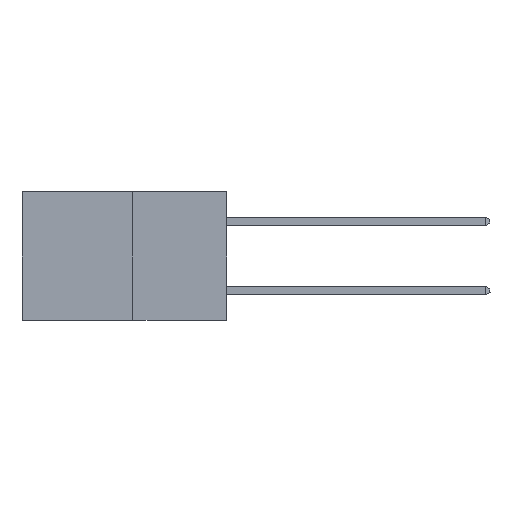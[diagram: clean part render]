
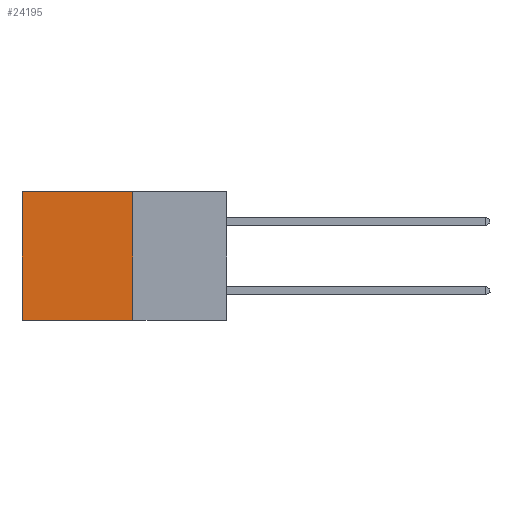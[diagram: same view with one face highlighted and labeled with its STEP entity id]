
A CAD part, left-side view. The second image highlights one B-rep face of the part: STEP entity #24195.
In plain terms, the highlighted planar face has unit normal (-1, 0, 0).
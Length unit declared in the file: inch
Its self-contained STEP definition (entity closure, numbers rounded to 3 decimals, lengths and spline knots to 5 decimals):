
#1287 = DIRECTION ( 'NONE',  ( 0., 0., -1. ) ) ;
#1591 = LINE ( 'NONE', #22627, #19816 ) ;
#2851 = CARTESIAN_POINT ( 'NONE',  ( 0.277, 0.59, -0.37 ) ) ;
#3229 = ORIENTED_EDGE ( 'NONE', *, *, #11312, .T. ) ;
#4168 = EDGE_CURVE ( 'NONE', #6265, #18495, #6261, .T. ) ;
#4348 = VECTOR ( 'NONE', #26284, 39.37008 ) ;
#5736 = EDGE_CURVE ( 'NONE', #10823, #8183, #19189, .T. ) ;
#6095 = CARTESIAN_POINT ( 'NONE',  ( 0.277, 0.27, -0.37 ) ) ;
#6261 = LINE ( 'NONE', #18632, #24426 ) ;
#6265 = VERTEX_POINT ( 'NONE', #29630 ) ;
#6326 = DIRECTION ( 'NONE',  ( 0., 0., -1. ) ) ;
#7198 = ORIENTED_EDGE ( 'NONE', *, *, #19954, .F. ) ;
#8137 = CARTESIAN_POINT ( 'NONE',  ( 0.277, 0.27, -0.37 ) ) ;
#8183 = VERTEX_POINT ( 'NONE', #8137 ) ;
#8268 = PLANE ( 'NONE',  #19540 ) ;
#8365 = CARTESIAN_POINT ( 'NONE',  ( 0.277, 0.27, -0.37 ) ) ;
#9035 = ORIENTED_EDGE ( 'NONE', *, *, #4168, .T. ) ;
#9748 = CARTESIAN_POINT ( 'NONE',  ( 0.277, 0.27, 0. ) ) ;
#10823 = VERTEX_POINT ( 'NONE', #26926 ) ;
#11312 = EDGE_CURVE ( 'NONE', #10823, #6265, #28799, .T. ) ;
#13213 = FACE_OUTER_BOUND ( 'NONE', #18186, .T. ) ;
#15457 = DIRECTION ( 'NONE',  ( 1., 0., 0. ) ) ;
#18186 = EDGE_LOOP ( 'NONE', ( #9035, #7198, #27432, #3229 ) ) ;
#18495 = VERTEX_POINT ( 'NONE', #2851 ) ;
#18632 = CARTESIAN_POINT ( 'NONE',  ( 0.277, 0.59, -0.37 ) ) ;
#19189 = LINE ( 'NONE', #6095, #25430 ) ;
#19540 = AXIS2_PLACEMENT_3D ( 'NONE', #8365, #15457, #1287 ) ;
#19816 = VECTOR ( 'NONE', #24985, 39.37008 ) ;
#19954 = EDGE_CURVE ( 'NONE', #8183, #18495, #1591, .T. ) ;
#22627 = CARTESIAN_POINT ( 'NONE',  ( 0.277, 0.27, -0.37 ) ) ;
#24195 = ADVANCED_FACE ( 'NONE', ( #13213 ), #8268, .F. ) ;
#24426 = VECTOR ( 'NONE', #24473, 39.37008 ) ;
#24473 = DIRECTION ( 'NONE',  ( 0., 0., -1. ) ) ;
#24985 = DIRECTION ( 'NONE',  ( 0., 1., 0. ) ) ;
#25430 = VECTOR ( 'NONE', #6326, 39.37008 ) ;
#26284 = DIRECTION ( 'NONE',  ( 0., 1., 0. ) ) ;
#26926 = CARTESIAN_POINT ( 'NONE',  ( 0.277, 0.27, 0. ) ) ;
#27432 = ORIENTED_EDGE ( 'NONE', *, *, #5736, .F. ) ;
#28799 = LINE ( 'NONE', #9748, #4348 ) ;
#29630 = CARTESIAN_POINT ( 'NONE',  ( 0.277, 0.59, 0. ) ) ;
